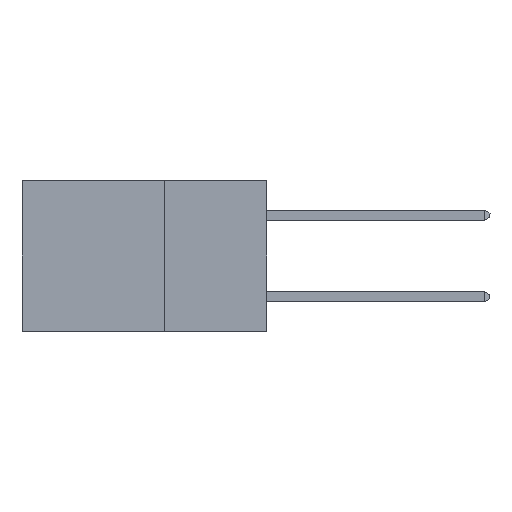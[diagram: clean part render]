
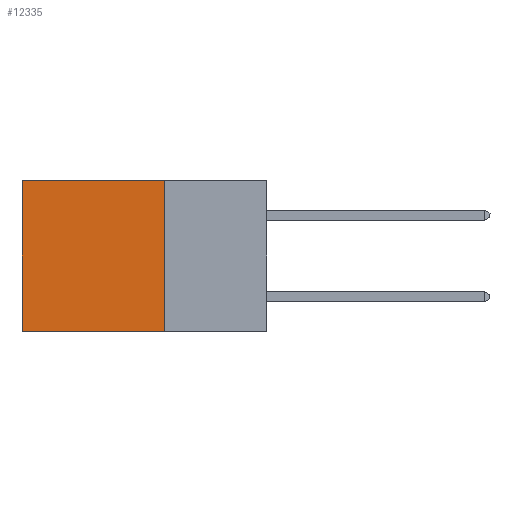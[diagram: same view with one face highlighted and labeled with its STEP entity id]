
A CAD part, left-side view. The second image highlights one B-rep face of the part: STEP entity #12335.
In plain terms, the highlighted planar face has unit normal (-1, 0, 0).
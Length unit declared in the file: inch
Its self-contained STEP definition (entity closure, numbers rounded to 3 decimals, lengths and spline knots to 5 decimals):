
#133 = DIRECTION ( 'NONE',  ( 0., 0., -1. ) ) ;
#1008 = ORIENTED_EDGE ( 'NONE', *, *, #7778, .T. ) ;
#1337 = VECTOR ( 'NONE', #13038, 39.37008 ) ;
#1522 = DIRECTION ( 'NONE',  ( 0., 0., -1. ) ) ;
#1739 = AXIS2_PLACEMENT_3D ( 'NONE', #3311, #12333, #5643 ) ;
#1844 = ORIENTED_EDGE ( 'NONE', *, *, #11920, .T. ) ;
#1999 = CARTESIAN_POINT ( 'NONE',  ( 0.2875, 0.6, -0.37 ) ) ;
#2084 = PLANE ( 'NONE',  #1739 ) ;
#2474 = FACE_OUTER_BOUND ( 'NONE', #12178, .T. ) ;
#2910 = LINE ( 'NONE', #9629, #14363 ) ;
#3218 = ORIENTED_EDGE ( 'NONE', *, *, #7192, .F. ) ;
#3311 = CARTESIAN_POINT ( 'NONE',  ( 0.2875, 0.25, 0. ) ) ;
#3856 = LINE ( 'NONE', #13787, #6928 ) ;
#5108 = CARTESIAN_POINT ( 'NONE',  ( 0.2875, 0.25, 0. ) ) ;
#5643 = DIRECTION ( 'NONE',  ( 0., 0., -1. ) ) ;
#6067 = ORIENTED_EDGE ( 'NONE', *, *, #8679, .F. ) ;
#6928 = VECTOR ( 'NONE', #133, 39.37008 ) ;
#7020 = VERTEX_POINT ( 'NONE', #9393 ) ;
#7192 = EDGE_CURVE ( 'NONE', #12120, #12702, #2910, .T. ) ;
#7778 = EDGE_CURVE ( 'NONE', #7020, #10175, #3856, .T. ) ;
#8481 = CARTESIAN_POINT ( 'NONE',  ( 0.2875, 0.25, -0.37 ) ) ;
#8679 = EDGE_CURVE ( 'NONE', #12702, #10175, #13359, .T. ) ;
#8712 = VECTOR ( 'NONE', #11580, 39.37008 ) ;
#8792 = CARTESIAN_POINT ( 'NONE',  ( 0.2875, 0.25, -0.37 ) ) ;
#9393 = CARTESIAN_POINT ( 'NONE',  ( 0.2875, 0.6, 0. ) ) ;
#9409 = LINE ( 'NONE', #13580, #8712 ) ;
#9629 = CARTESIAN_POINT ( 'NONE',  ( 0.2875, 0.25, 0. ) ) ;
#10175 = VERTEX_POINT ( 'NONE', #1999 ) ;
#11580 = DIRECTION ( 'NONE',  ( 0., 1., 0. ) ) ;
#11920 = EDGE_CURVE ( 'NONE', #12120, #7020, #9409, .T. ) ;
#12120 = VERTEX_POINT ( 'NONE', #5108 ) ;
#12178 = EDGE_LOOP ( 'NONE', ( #1008, #6067, #3218, #1844 ) ) ;
#12333 = DIRECTION ( 'NONE',  ( 1., 0., 0. ) ) ;
#12335 = ADVANCED_FACE ( 'NONE', ( #2474 ), #2084, .F. ) ;
#12702 = VERTEX_POINT ( 'NONE', #8481 ) ;
#13038 = DIRECTION ( 'NONE',  ( 0., 1., 0. ) ) ;
#13359 = LINE ( 'NONE', #8792, #1337 ) ;
#13580 = CARTESIAN_POINT ( 'NONE',  ( 0.2875, 0.25, 0. ) ) ;
#13787 = CARTESIAN_POINT ( 'NONE',  ( 0.2875, 0.6, 0. ) ) ;
#14363 = VECTOR ( 'NONE', #1522, 39.37008 ) ;
